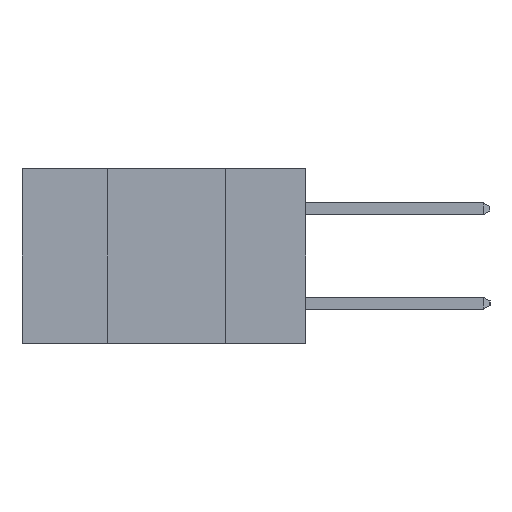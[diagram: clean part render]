
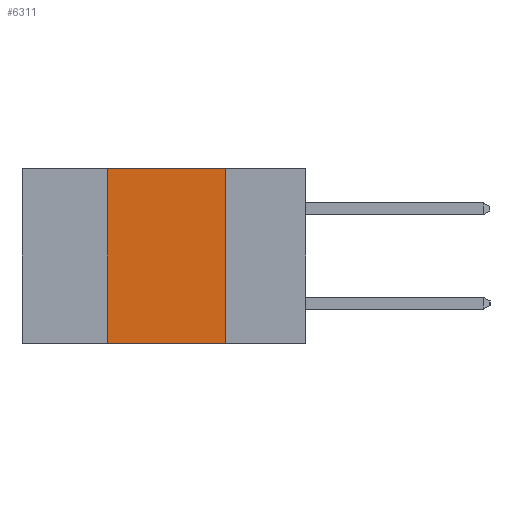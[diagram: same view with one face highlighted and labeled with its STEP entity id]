
A CAD part, left-side view. The second image highlights one B-rep face of the part: STEP entity #6311.
In plain terms, the highlighted planar face has unit normal (-1, 0, 0).
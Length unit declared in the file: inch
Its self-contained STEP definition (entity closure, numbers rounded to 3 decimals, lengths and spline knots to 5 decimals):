
#499 = CARTESIAN_POINT ( 'NONE',  ( 0., 0.17, -0.37 ) ) ;
#1173 = CARTESIAN_POINT ( 'NONE',  ( 0., 0.17, -0.37 ) ) ;
#1476 = VECTOR ( 'NONE', #10236, 39.37008 ) ;
#1645 = EDGE_CURVE ( 'NONE', #3084, #11617, #10986, .T. ) ;
#1773 = ORIENTED_EDGE ( 'NONE', *, *, #14146, .T. ) ;
#2110 = DIRECTION ( 'NONE',  ( 0., -1., 0. ) ) ;
#2325 = VECTOR ( 'NONE', #2110, 39.37008 ) ;
#2643 = CARTESIAN_POINT ( 'NONE',  ( 0., 0.42, -0.37 ) ) ;
#2992 = DIRECTION ( 'NONE',  ( 1., 0., 0. ) ) ;
#3021 = ORIENTED_EDGE ( 'NONE', *, *, #1645, .F. ) ;
#3084 = VERTEX_POINT ( 'NONE', #2643 ) ;
#3166 = VERTEX_POINT ( 'NONE', #499 ) ;
#3457 = PLANE ( 'NONE',  #4019 ) ;
#3529 = DIRECTION ( 'NONE',  ( 0., 0., -1. ) ) ;
#3834 = CARTESIAN_POINT ( 'NONE',  ( 0., 0.6, 0. ) ) ;
#3970 = ORIENTED_EDGE ( 'NONE', *, *, #12176, .F. ) ;
#4019 = AXIS2_PLACEMENT_3D ( 'NONE', #3834, #2992, #3529 ) ;
#4055 = ORIENTED_EDGE ( 'NONE', *, *, #13644, .F. ) ;
#4237 = DIRECTION ( 'NONE',  ( 0., -1., 0. ) ) ;
#6121 = FACE_OUTER_BOUND ( 'NONE', #12010, .T. ) ;
#6311 = ADVANCED_FACE ( 'NONE', ( #6121 ), #3457, .F. ) ;
#6641 = DIRECTION ( 'NONE',  ( 0., 0., 1. ) ) ;
#6751 = LINE ( 'NONE', #1173, #1476 ) ;
#6857 = CARTESIAN_POINT ( 'NONE',  ( 0., 0.42, -0.37 ) ) ;
#7817 = CARTESIAN_POINT ( 'NONE',  ( 0., 0.17, 0. ) ) ;
#7971 = VECTOR ( 'NONE', #6641, 39.37008 ) ;
#8884 = CARTESIAN_POINT ( 'NONE',  ( 0., 0.6, -0.37 ) ) ;
#9002 = CARTESIAN_POINT ( 'NONE',  ( 0., 0.42, 0. ) ) ;
#9680 = LINE ( 'NONE', #9895, #12234 ) ;
#9895 = CARTESIAN_POINT ( 'NONE',  ( 0., 0.6, 0. ) ) ;
#10236 = DIRECTION ( 'NONE',  ( 0., 0., -1. ) ) ;
#10986 = LINE ( 'NONE', #6857, #7971 ) ;
#11617 = VERTEX_POINT ( 'NONE', #9002 ) ;
#12010 = EDGE_LOOP ( 'NONE', ( #4055, #3970, #3021, #1773 ) ) ;
#12176 = EDGE_CURVE ( 'NONE', #11617, #14201, #9680, .T. ) ;
#12234 = VECTOR ( 'NONE', #4237, 39.37008 ) ;
#13644 = EDGE_CURVE ( 'NONE', #14201, #3166, #6751, .T. ) ;
#13863 = LINE ( 'NONE', #8884, #2325 ) ;
#14146 = EDGE_CURVE ( 'NONE', #3084, #3166, #13863, .T. ) ;
#14201 = VERTEX_POINT ( 'NONE', #7817 ) ;
